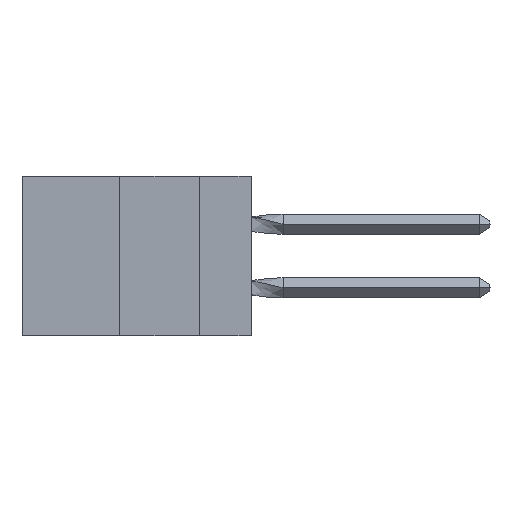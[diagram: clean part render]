
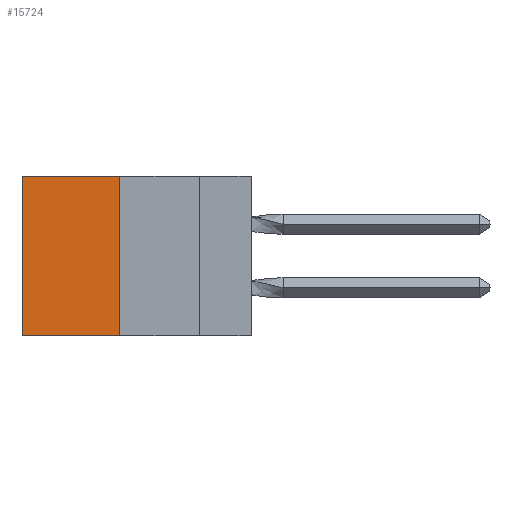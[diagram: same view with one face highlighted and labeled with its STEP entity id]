
A CAD part, left-side view. The second image highlights one B-rep face of the part: STEP entity #15724.
In plain terms, the highlighted planar face has unit normal (-1, 0, 0).
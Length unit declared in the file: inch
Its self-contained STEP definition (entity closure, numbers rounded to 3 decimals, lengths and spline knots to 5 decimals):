
#388 = CARTESIAN_POINT ( 'NONE',  ( 0.305, 0.413, -0.5 ) ) ;
#1548 = ORIENTED_EDGE ( 'NONE', *, *, #8715, .T. ) ;
#2365 = EDGE_CURVE ( 'NONE', #11978, #2920, #12935, .T. ) ;
#2920 = VERTEX_POINT ( 'NONE', #15512 ) ;
#3575 = ORIENTED_EDGE ( 'NONE', *, *, #2365, .T. ) ;
#4093 = CARTESIAN_POINT ( 'NONE',  ( 0.305, 0.413, -0.5 ) ) ;
#4135 = CARTESIAN_POINT ( 'NONE',  ( 0.305, 0.72, -0.5 ) ) ;
#4226 = CARTESIAN_POINT ( 'NONE',  ( 0.305, 0.413, 0. ) ) ;
#4842 = VERTEX_POINT ( 'NONE', #10131 ) ;
#5050 = CARTESIAN_POINT ( 'NONE',  ( 0.305, 0.413, -0.5 ) ) ;
#5949 = AXIS2_PLACEMENT_3D ( 'NONE', #5050, #13964, #8894 ) ;
#7138 = EDGE_CURVE ( 'NONE', #4842, #9030, #14846, .T. ) ;
#7159 = EDGE_CURVE ( 'NONE', #11978, #4842, #11742, .T. ) ;
#7610 = PLANE ( 'NONE',  #5949 ) ;
#7883 = DIRECTION ( 'NONE',  ( 0., 0., -1. ) ) ;
#8632 = FACE_OUTER_BOUND ( 'NONE', #11566, .T. ) ;
#8715 = EDGE_CURVE ( 'NONE', #2920, #9030, #13081, .T. ) ;
#8894 = DIRECTION ( 'NONE',  ( 0., 0., -1. ) ) ;
#9030 = VERTEX_POINT ( 'NONE', #4135 ) ;
#10131 = CARTESIAN_POINT ( 'NONE',  ( 0.305, 0.413, -0.5 ) ) ;
#10337 = CARTESIAN_POINT ( 'NONE',  ( 0.305, 0.72, -0.5 ) ) ;
#10488 = VECTOR ( 'NONE', #7883, 39.37008 ) ;
#10641 = ORIENTED_EDGE ( 'NONE', *, *, #7159, .F. ) ;
#10910 = VECTOR ( 'NONE', #14435, 39.37008 ) ;
#11313 = VECTOR ( 'NONE', #13013, 39.37008 ) ;
#11566 = EDGE_LOOP ( 'NONE', ( #1548, #12686, #10641, #3575 ) ) ;
#11742 = LINE ( 'NONE', #4093, #11313 ) ;
#11978 = VERTEX_POINT ( 'NONE', #15354 ) ;
#12686 = ORIENTED_EDGE ( 'NONE', *, *, #7138, .F. ) ;
#12935 = LINE ( 'NONE', #4226, #13143 ) ;
#13013 = DIRECTION ( 'NONE',  ( 0., 0., -1. ) ) ;
#13081 = LINE ( 'NONE', #10337, #10488 ) ;
#13091 = DIRECTION ( 'NONE',  ( 0., 1., 0. ) ) ;
#13143 = VECTOR ( 'NONE', #13091, 39.37008 ) ;
#13964 = DIRECTION ( 'NONE',  ( 1., 0., 0. ) ) ;
#14435 = DIRECTION ( 'NONE',  ( 0., 1., 0. ) ) ;
#14846 = LINE ( 'NONE', #388, #10910 ) ;
#15354 = CARTESIAN_POINT ( 'NONE',  ( 0.305, 0.413, 0. ) ) ;
#15512 = CARTESIAN_POINT ( 'NONE',  ( 0.305, 0.72, 0. ) ) ;
#15724 = ADVANCED_FACE ( 'NONE', ( #8632 ), #7610, .F. ) ;
